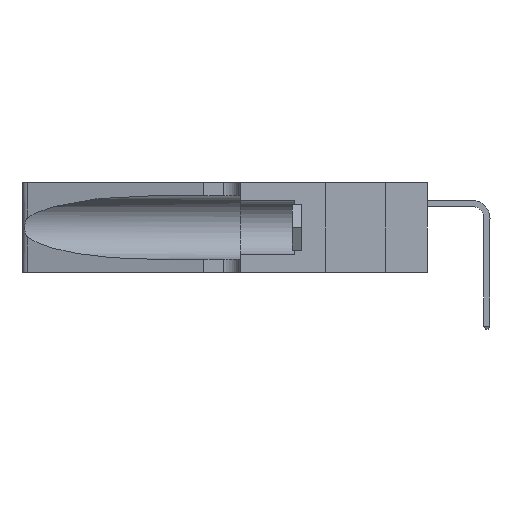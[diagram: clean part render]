
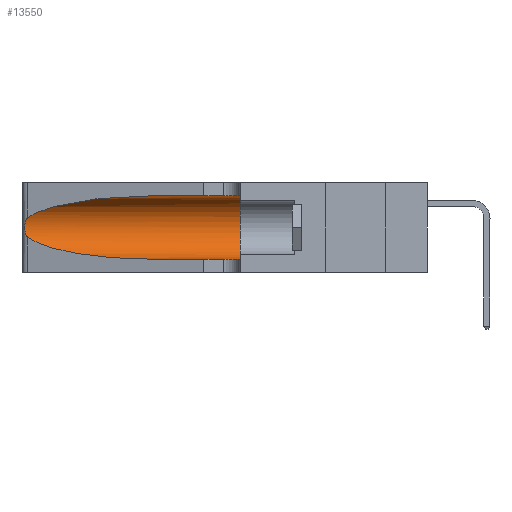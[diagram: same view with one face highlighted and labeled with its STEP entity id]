
A CAD part, left-side view. The second image highlights one B-rep face of the part: STEP entity #13550.
In plain terms, the highlighted cylindrical face has radius 3.308 mm (diameter 6.617 mm), a partial arc.
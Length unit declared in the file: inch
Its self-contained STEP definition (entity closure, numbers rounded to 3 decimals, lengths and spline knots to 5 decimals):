
#141 = CARTESIAN_POINT ( 'NONE',  ( 0.26075, 1.23896, 0.19203 ) ) ;
#252 = ORIENTED_EDGE ( 'NONE', *, *, #11204, .T. ) ;
#1597 = EDGE_CURVE ( 'NONE', #9649, #17534, #21398, .T. ) ;
#1872 = DIRECTION ( 'NONE',  ( 0., 1., 0. ) ) ;
#1878 = CARTESIAN_POINT ( 'NONE',  ( 0.25487, 1.22718, 0.14631 ) ) ;
#2423 = CARTESIAN_POINT ( 'NONE',  ( 0.26017, 1.23833, 0.17102 ) ) ;
#4144 = EDGE_CURVE ( 'NONE', #17609, #4654, #6098, .T. ) ;
#4278 = CARTESIAN_POINT ( 'NONE',  ( 0.18966, 0.96281, 0.31525 ) ) ;
#4654 = VERTEX_POINT ( 'NONE', #23978 ) ;
#4727 = CARTESIAN_POINT ( 'NONE',  ( 0.25789, 1.23486, 0.15765 ) ) ;
#4873 = CARTESIAN_POINT ( 'NONE',  ( 0.1305, 0.35, 0.05475 ) ) ;
#5250 = DIRECTION ( 'NONE',  ( 0., 0., -1. ) ) ;
#5346 = DIRECTION ( 'NONE',  ( 0., -1., 0. ) ) ;
#6098 = B_SPLINE_CURVE_WITH_KNOTS ( 'NONE', 3,
 ( #24294, #24198, #21985, #11278, #26465, #13448, #141, #15658, #2423, #17794, #4727, #19966, #6929, #22183 ),
 .UNSPECIFIED., .F., .F.,
 ( 4, 2, 2, 2, 2, 2, 4 ),
 ( 0., 0.00027, 0.00053, 0.00107, 0.0016, 0.00187, 0.00214 ),
 .UNSPECIFIED. ) ;
#6411 = CARTESIAN_POINT ( 'NONE',  ( 0.18966, 0.96281, 0.05475 ) ) ;
#6929 = CARTESIAN_POINT ( 'NONE',  ( 0.25555, 1.22993, 0.14849 ) ) ;
#7868 = ORIENTED_EDGE ( 'NONE', *, *, #1597, .F. ) ;
#8991 = VERTEX_POINT ( 'NONE', #11130 ) ;
#9649 = VERTEX_POINT ( 'NONE', #22106 ) ;
#10787 = EDGE_CURVE ( 'NONE', #9649, #17609, #19174, .T. ) ;
#10945 = CARTESIAN_POINT ( 'NONE',  ( 0.25487, 1.22718, 0.22369 ) ) ;
#10949 = VERTEX_POINT ( 'NONE', #4873 ) ;
#11121 = ORIENTED_EDGE ( 'NONE', *, *, #4144, .T. ) ;
#11130 = CARTESIAN_POINT ( 'NONE',  ( 0.1305, 0.72297, 0.05475 ) ) ;
#11204 = EDGE_CURVE ( 'NONE', #8991, #10949, #18673, .T. ) ;
#11278 = CARTESIAN_POINT ( 'NONE',  ( 0.25787, 1.23484, 0.2124 ) ) ;
#11778 = FACE_OUTER_BOUND ( 'NONE', #27350, .T. ) ;
#11879 = CARTESIAN_POINT ( 'NONE',  ( 0.1305, 1.61858, 0.185 ) ) ;
#12945 = VECTOR ( 'NONE', #25358, 39.37008 ) ;
#13448 = CARTESIAN_POINT ( 'NONE',  ( 0.26018, 1.23835, 0.19895 ) ) ;
#13550 = ADVANCED_FACE ( 'NONE', ( #11778 ), #22640, .F. ) ;
#14687 = ORIENTED_EDGE ( 'NONE', *, *, #26268, .F. ) ;
#15130 = CARTESIAN_POINT ( 'NONE',  ( 0.1305, 0.35, 0.185 ) ) ;
#15240 = CARTESIAN_POINT ( 'NONE',  ( 0.1305, 0.72297, 0.31525 ) ) ;
#15645 = VECTOR ( 'NONE', #23979, 39.37008 ) ;
#15658 = CARTESIAN_POINT ( 'NONE',  ( 0.26075, 1.23896, 0.178 ) ) ;
#16734 = ORIENTED_EDGE ( 'NONE', *, *, #10787, .T. ) ;
#17277 = DIRECTION ( 'NONE',  ( 0., 0., 1. ) ) ;
#17534 = VERTEX_POINT ( 'NONE', #22583 ) ;
#17609 = VERTEX_POINT ( 'NONE', #22871 ) ;
#17794 = CARTESIAN_POINT ( 'NONE',  ( 0.25856, 1.23593, 0.16098 ) ) ;
#18202 = CIRCLE ( 'NONE', #20504, 0.13025 ) ;
#18673 = LINE ( 'NONE', #18755, #12945 ) ;
#18755 = CARTESIAN_POINT ( 'NONE',  ( 0.1305, 1.61858, 0.05475 ) ) ;
#19116 = EDGE_CURVE ( 'NONE', #4654, #8991, #27206, .T. ) ;
#19174 =( BOUNDED_CURVE ( )  B_SPLINE_CURVE ( 3, ( #15240, #4278, #23963, #10945 ),
 .UNSPECIFIED., .F., .T. ) 
 B_SPLINE_CURVE_WITH_KNOTS ( ( 4, 4 ),
 ( 1.5708, 2.84003 ),
 .UNSPECIFIED. ) 
 CURVE ( )  GEOMETRIC_REPRESENTATION_ITEM ( )  RATIONAL_B_SPLINE_CURVE ( ( 1., 0.87, 0.87, 1. ) ) 
 REPRESENTATION_ITEM ( '' )  );
#19434 = CARTESIAN_POINT ( 'NONE',  ( 0.2373, 1.15595, 0.08982 ) ) ;
#19966 = CARTESIAN_POINT ( 'NONE',  ( 0.25639, 1.23186, 0.15144 ) ) ;
#20504 = AXIS2_PLACEMENT_3D ( 'NONE', #15130, #1872, #17277 ) ;
#21398 = LINE ( 'NONE', #24046, #15645 ) ;
#21640 = CARTESIAN_POINT ( 'NONE',  ( 0.1305, 0.72297, 0.05475 ) ) ;
#21985 = CARTESIAN_POINT ( 'NONE',  ( 0.25639, 1.23184, 0.21858 ) ) ;
#22106 = CARTESIAN_POINT ( 'NONE',  ( 0.1305, 0.72297, 0.31525 ) ) ;
#22183 = CARTESIAN_POINT ( 'NONE',  ( 0.25487, 1.22718, 0.14631 ) ) ;
#22583 = CARTESIAN_POINT ( 'NONE',  ( 0.1305, 0.35, 0.31525 ) ) ;
#22640 = CYLINDRICAL_SURFACE ( 'NONE', #28121, 0.13025 ) ;
#22871 = CARTESIAN_POINT ( 'NONE',  ( 0.25487, 1.22718, 0.22369 ) ) ;
#23963 = CARTESIAN_POINT ( 'NONE',  ( 0.2373, 1.15595, 0.28018 ) ) ;
#23978 = CARTESIAN_POINT ( 'NONE',  ( 0.25487, 1.22718, 0.14631 ) ) ;
#23979 = DIRECTION ( 'NONE',  ( 0., -1., 0. ) ) ;
#24046 = CARTESIAN_POINT ( 'NONE',  ( 0.1305, 1.61858, 0.31525 ) ) ;
#24198 = CARTESIAN_POINT ( 'NONE',  ( 0.25555, 1.22994, 0.2215 ) ) ;
#24294 = CARTESIAN_POINT ( 'NONE',  ( 0.25487, 1.22718, 0.22369 ) ) ;
#25358 = DIRECTION ( 'NONE',  ( 0., -1., 0. ) ) ;
#26268 = EDGE_CURVE ( 'NONE', #17534, #10949, #18202, .T. ) ;
#26465 = CARTESIAN_POINT ( 'NONE',  ( 0.25854, 1.2359, 0.20912 ) ) ;
#26809 = ORIENTED_EDGE ( 'NONE', *, *, #19116, .T. ) ;
#27206 =( BOUNDED_CURVE ( )  B_SPLINE_CURVE ( 3, ( #1878, #19434, #6411, #21640 ),
 .UNSPECIFIED., .F., .F. ) 
 B_SPLINE_CURVE_WITH_KNOTS ( ( 4, 4 ),
 ( 3.44316, 4.71239 ),
 .UNSPECIFIED. ) 
 CURVE ( )  GEOMETRIC_REPRESENTATION_ITEM ( )  RATIONAL_B_SPLINE_CURVE ( ( 1., 0.87, 0.87, 1. ) ) 
 REPRESENTATION_ITEM ( '' )  );
#27350 = EDGE_LOOP ( 'NONE', ( #16734, #11121, #26809, #252, #14687, #7868 ) ) ;
#28121 = AXIS2_PLACEMENT_3D ( 'NONE', #11879, #5346, #5250 ) ;
